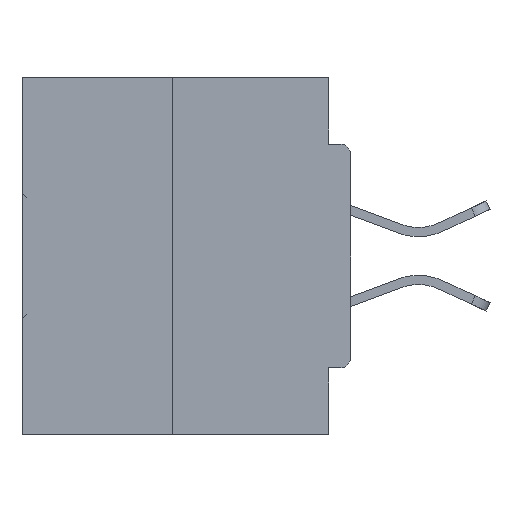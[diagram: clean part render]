
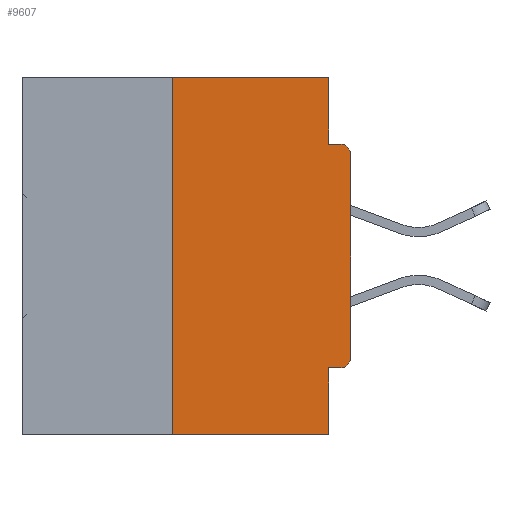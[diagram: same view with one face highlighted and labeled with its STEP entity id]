
A CAD part, left-side view. The second image highlights one B-rep face of the part: STEP entity #9607.
In plain terms, the highlighted planar face has unit normal (-1, 0, 0).
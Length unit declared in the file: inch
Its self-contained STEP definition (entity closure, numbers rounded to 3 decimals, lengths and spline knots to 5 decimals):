
#64 = DIRECTION ( 'NONE',  ( 0., 1., 0. ) ) ;
#66 = CARTESIAN_POINT ( 'NONE',  ( 0., 0.015, -0.1085 ) ) ;
#1163 = DIRECTION ( 'NONE',  ( 0., 0., 1. ) ) ;
#1624 = VERTEX_POINT ( 'NONE', #7542 ) ;
#1727 = CARTESIAN_POINT ( 'NONE',  ( 0., 0.015, -0.4065 ) ) ;
#3115 = VERTEX_POINT ( 'NONE', #12337 ) ;
#3407 = VERTEX_POINT ( 'NONE', #28101 ) ;
#3418 = CARTESIAN_POINT ( 'NONE',  ( 0., 0., 0. ) ) ;
#4169 = ORIENTED_EDGE ( 'NONE', *, *, #6784, .T. ) ;
#5395 = ORIENTED_EDGE ( 'NONE', *, *, #29755, .F. ) ;
#5694 = LINE ( 'NONE', #33061, #41897 ) ;
#6784 = EDGE_CURVE ( 'NONE', #22415, #1624, #32196, .T. ) ;
#7357 = DIRECTION ( 'NONE',  ( 0., 0., -1. ) ) ;
#7542 = CARTESIAN_POINT ( 'NONE',  ( 0., 0., -0.1085 ) ) ;
#8373 = PLANE ( 'NONE',  #41508 ) ;
#8465 = CARTESIAN_POINT ( 'NONE',  ( 0., 0.25, 0. ) ) ;
#8525 = DIRECTION ( 'NONE',  ( 1., 0., 0. ) ) ;
#9366 = EDGE_CURVE ( 'NONE', #13011, #22415, #27227, .T. ) ;
#9607 = ADVANCED_FACE ( 'NONE', ( #26630 ), #8373, .F. ) ;
#11671 = LINE ( 'NONE', #46701, #16174 ) ;
#12337 = CARTESIAN_POINT ( 'NONE',  ( 0., 0.031, 0. ) ) ;
#12707 = VERTEX_POINT ( 'NONE', #32431 ) ;
#13011 = VERTEX_POINT ( 'NONE', #1727 ) ;
#13385 = ORIENTED_EDGE ( 'NONE', *, *, #46891, .F. ) ;
#13457 = LINE ( 'NONE', #21415, #36619 ) ;
#14762 = ORIENTED_EDGE ( 'NONE', *, *, #15290, .F. ) ;
#15290 = EDGE_CURVE ( 'NONE', #12707, #21277, #36537, .T. ) ;
#15625 = CIRCLE ( 'NONE', #23844, 0.015 ) ;
#16174 = VECTOR ( 'NONE', #20911, 39.37008 ) ;
#16179 = VECTOR ( 'NONE', #1163, 39.37008 ) ;
#17235 = LINE ( 'NONE', #35708, #26844 ) ;
#17540 = DIRECTION ( 'NONE',  ( 0., -1., 0. ) ) ;
#17841 = DIRECTION ( 'NONE',  ( 0., 0., -1. ) ) ;
#20529 = DIRECTION ( 'NONE',  ( 0., 0., -1. ) ) ;
#20911 = DIRECTION ( 'NONE',  ( 0., -1., 0. ) ) ;
#21178 = ORIENTED_EDGE ( 'NONE', *, *, #46855, .T. ) ;
#21277 = VERTEX_POINT ( 'NONE', #44384 ) ;
#21415 = CARTESIAN_POINT ( 'NONE',  ( 0., 0., -0.4065 ) ) ;
#22415 = VERTEX_POINT ( 'NONE', #35269 ) ;
#22653 = LINE ( 'NONE', #29850, #43041 ) ;
#23220 = CARTESIAN_POINT ( 'NONE',  ( 0., 0.031, -0.5 ) ) ;
#23844 = AXIS2_PLACEMENT_3D ( 'NONE', #66, #25373, #7357 ) ;
#25113 = DIRECTION ( 'NONE',  ( -1., 0., 0. ) ) ;
#25277 = CARTESIAN_POINT ( 'NONE',  ( 0., 0.015, -0.3915 ) ) ;
#25373 = DIRECTION ( 'NONE',  ( -1., 0., 0. ) ) ;
#26077 = DIRECTION ( 'NONE',  ( 0., -1., 0. ) ) ;
#26630 = FACE_OUTER_BOUND ( 'NONE', #44881, .T. ) ;
#26844 = VECTOR ( 'NONE', #17540, 39.37008 ) ;
#27227 = CIRCLE ( 'NONE', #32426, 0.015 ) ;
#27647 = VECTOR ( 'NONE', #20529, 39.37008 ) ;
#28101 = CARTESIAN_POINT ( 'NONE',  ( 0., 0.031, -0.5 ) ) ;
#29063 = EDGE_CURVE ( 'NONE', #42982, #3407, #37238, .T. ) ;
#29199 = DIRECTION ( 'NONE',  ( 0., 0., 1. ) ) ;
#29755 = EDGE_CURVE ( 'NONE', #13011, #42982, #13457, .T. ) ;
#29850 = CARTESIAN_POINT ( 'NONE',  ( 0., 0.031, 0. ) ) ;
#30765 = DIRECTION ( 'NONE',  ( 0., 0., -1. ) ) ;
#31389 = VERTEX_POINT ( 'NONE', #36656 ) ;
#32196 = LINE ( 'NONE', #3418, #46363 ) ;
#32426 = AXIS2_PLACEMENT_3D ( 'NONE', #25277, #25113, #17841 ) ;
#32431 = CARTESIAN_POINT ( 'NONE',  ( 0., 0.25, -0.5 ) ) ;
#33061 = CARTESIAN_POINT ( 'NONE',  ( 0., 0.46, -0.5 ) ) ;
#33340 = CARTESIAN_POINT ( 'NONE',  ( 0., 0.46, 0. ) ) ;
#34193 = CARTESIAN_POINT ( 'NONE',  ( 0., 0.031, -0.0935 ) ) ;
#34518 = EDGE_CURVE ( 'NONE', #21277, #3115, #11671, .T. ) ;
#35141 = EDGE_CURVE ( 'NONE', #43101, #31389, #17235, .T. ) ;
#35269 = CARTESIAN_POINT ( 'NONE',  ( 0., 0., -0.3915 ) ) ;
#35708 = CARTESIAN_POINT ( 'NONE',  ( 0., 0., -0.0935 ) ) ;
#36537 = LINE ( 'NONE', #8465, #16179 ) ;
#36619 = VECTOR ( 'NONE', #64, 39.37008 ) ;
#36656 = CARTESIAN_POINT ( 'NONE',  ( 0., 0.015, -0.0935 ) ) ;
#36870 = CARTESIAN_POINT ( 'NONE',  ( 0., 0.031, -0.4065 ) ) ;
#37238 = LINE ( 'NONE', #23220, #27647 ) ;
#37774 = ORIENTED_EDGE ( 'NONE', *, *, #29063, .F. ) ;
#38427 = ORIENTED_EDGE ( 'NONE', *, *, #42033, .T. ) ;
#38475 = ORIENTED_EDGE ( 'NONE', *, *, #9366, .T. ) ;
#41508 = AXIS2_PLACEMENT_3D ( 'NONE', #33340, #8525, #30765 ) ;
#41603 = ORIENTED_EDGE ( 'NONE', *, *, #35141, .F. ) ;
#41897 = VECTOR ( 'NONE', #26077, 39.37008 ) ;
#42033 = EDGE_CURVE ( 'NONE', #1624, #31389, #15625, .T. ) ;
#42982 = VERTEX_POINT ( 'NONE', #36870 ) ;
#43041 = VECTOR ( 'NONE', #45053, 39.37008 ) ;
#43101 = VERTEX_POINT ( 'NONE', #34193 ) ;
#43226 = ORIENTED_EDGE ( 'NONE', *, *, #34518, .F. ) ;
#44384 = CARTESIAN_POINT ( 'NONE',  ( 0., 0.25, 0. ) ) ;
#44881 = EDGE_LOOP ( 'NONE', ( #43226, #14762, #21178, #37774, #5395, #38475, #4169, #38427, #41603, #13385 ) ) ;
#45053 = DIRECTION ( 'NONE',  ( 0., 0., -1. ) ) ;
#46363 = VECTOR ( 'NONE', #29199, 39.37008 ) ;
#46701 = CARTESIAN_POINT ( 'NONE',  ( 0., 0.46, 0. ) ) ;
#46855 = EDGE_CURVE ( 'NONE', #12707, #3407, #5694, .T. ) ;
#46891 = EDGE_CURVE ( 'NONE', #3115, #43101, #22653, .T. ) ;
